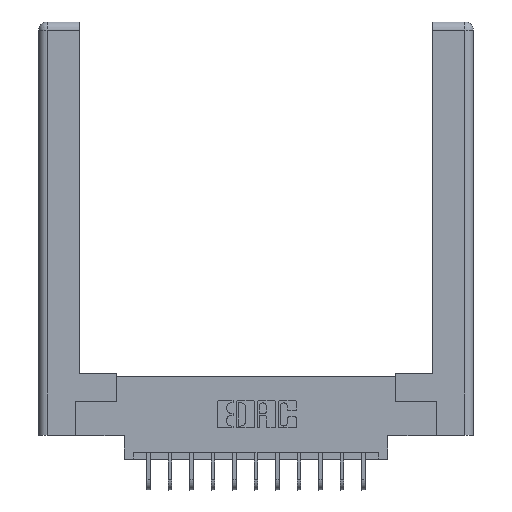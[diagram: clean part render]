
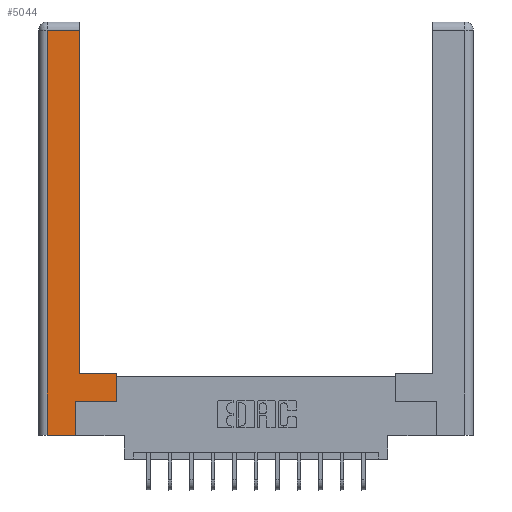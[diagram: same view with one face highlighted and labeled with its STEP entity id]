
A CAD part, top view. The second image highlights one B-rep face of the part: STEP entity #5044.
In plain terms, the highlighted planar face has unit normal (0, 0, 1).
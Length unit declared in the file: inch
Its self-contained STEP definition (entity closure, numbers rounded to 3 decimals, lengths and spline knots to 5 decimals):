
#71 = LINE ( 'NONE', #1686, #12676 ) ;
#264 = EDGE_CURVE ( 'NONE', #10003, #4532, #17100, .T. ) ;
#287 = EDGE_LOOP ( 'NONE', ( #3991, #10321, #2021, #16963, #15825, #12860, #7349, #15462 ) ) ;
#329 = DIRECTION ( 'NONE',  ( 1., 0., 0. ) ) ;
#395 = DIRECTION ( 'NONE',  ( 1., 0., 0. ) ) ;
#688 = VECTOR ( 'NONE', #10674, 39.37008 ) ;
#1391 = CARTESIAN_POINT ( 'NONE',  ( 0.0615, 0., 0. ) ) ;
#1444 = CARTESIAN_POINT ( 'NONE',  ( 0.265, 0.245, 0. ) ) ;
#1686 = CARTESIAN_POINT ( 'NONE',  ( 0.295, 0.45, 0. ) ) ;
#1974 = LINE ( 'NONE', #9517, #12900 ) ;
#2021 = ORIENTED_EDGE ( 'NONE', *, *, #264, .T. ) ;
#2896 = VERTEX_POINT ( 'NONE', #10960 ) ;
#2927 = EDGE_CURVE ( 'NONE', #10829, #9337, #16810, .T. ) ;
#3991 = ORIENTED_EDGE ( 'NONE', *, *, #9519, .T. ) ;
#4105 = VECTOR ( 'NONE', #11520, 39.37008 ) ;
#4425 = CARTESIAN_POINT ( 'NONE',  ( 0.0615, 2.94, 0. ) ) ;
#4426 = AXIS2_PLACEMENT_3D ( 'NONE', #12154, #8090, #5391 ) ;
#4532 = VERTEX_POINT ( 'NONE', #1391 ) ;
#4534 = LINE ( 'NONE', #4994, #4105 ) ;
#4980 = DIRECTION ( 'NONE',  ( -1., 0., 0. ) ) ;
#4994 = CARTESIAN_POINT ( 'NONE',  ( 0.295, 3., 0. ) ) ;
#5044 = ADVANCED_FACE ( 'NONE', ( #5774 ), #13354, .F. ) ;
#5070 = CARTESIAN_POINT ( 'NONE',  ( 0.265, 0.245, 0. ) ) ;
#5391 = DIRECTION ( 'NONE',  ( -1., 0., 0. ) ) ;
#5774 = FACE_OUTER_BOUND ( 'NONE', #287, .T. ) ;
#5861 = CARTESIAN_POINT ( 'NONE',  ( 0.295, 0.45, 0. ) ) ;
#7019 = VECTOR ( 'NONE', #4980, 39.37008 ) ;
#7349 = ORIENTED_EDGE ( 'NONE', *, *, #12414, .T. ) ;
#7910 = EDGE_CURVE ( 'NONE', #4532, #8687, #8053, .T. ) ;
#8053 = LINE ( 'NONE', #9429, #13867 ) ;
#8090 = DIRECTION ( 'NONE',  ( 0., 0., -1. ) ) ;
#8107 = CARTESIAN_POINT ( 'NONE',  ( 0.565, 0.245, 0. ) ) ;
#8336 = EDGE_CURVE ( 'NONE', #2896, #10003, #12626, .T. ) ;
#8687 = VERTEX_POINT ( 'NONE', #15212 ) ;
#8796 = VECTOR ( 'NONE', #10951, 39.37008 ) ;
#9337 = VERTEX_POINT ( 'NONE', #12752 ) ;
#9429 = CARTESIAN_POINT ( 'NONE',  ( 0.265, 0., 0. ) ) ;
#9517 = CARTESIAN_POINT ( 'NONE',  ( 0.565, 0.45, 0. ) ) ;
#9519 = EDGE_CURVE ( 'NONE', #13695, #2896, #4534, .T. ) ;
#9758 = VECTOR ( 'NONE', #395, 39.37008 ) ;
#10003 = VERTEX_POINT ( 'NONE', #4425 ) ;
#10321 = ORIENTED_EDGE ( 'NONE', *, *, #8336, .T. ) ;
#10674 = DIRECTION ( 'NONE',  ( 0., 1., 0. ) ) ;
#10829 = VERTEX_POINT ( 'NONE', #5070 ) ;
#10951 = DIRECTION ( 'NONE',  ( 0., -1., 0. ) ) ;
#10960 = CARTESIAN_POINT ( 'NONE',  ( 0.295, 2.94, 0. ) ) ;
#11065 = CARTESIAN_POINT ( 'NONE',  ( 0.0615, 0., 0. ) ) ;
#11443 = VERTEX_POINT ( 'NONE', #13850 ) ;
#11520 = DIRECTION ( 'NONE',  ( 0., 1., 0. ) ) ;
#12154 = CARTESIAN_POINT ( 'NONE',  ( 0., 0., 0. ) ) ;
#12233 = DIRECTION ( 'NONE',  ( -1., 0., 0. ) ) ;
#12414 = EDGE_CURVE ( 'NONE', #9337, #11443, #1974, .T. ) ;
#12626 = LINE ( 'NONE', #14305, #7019 ) ;
#12676 = VECTOR ( 'NONE', #12233, 39.37008 ) ;
#12752 = CARTESIAN_POINT ( 'NONE',  ( 0.565, 0.245, 0. ) ) ;
#12860 = ORIENTED_EDGE ( 'NONE', *, *, #2927, .T. ) ;
#12900 = VECTOR ( 'NONE', #14870, 39.37008 ) ;
#13077 = EDGE_CURVE ( 'NONE', #11443, #13695, #71, .T. ) ;
#13354 = PLANE ( 'NONE',  #4426 ) ;
#13695 = VERTEX_POINT ( 'NONE', #5861 ) ;
#13850 = CARTESIAN_POINT ( 'NONE',  ( 0.565, 0.45, 0. ) ) ;
#13867 = VECTOR ( 'NONE', #329, 39.37008 ) ;
#14305 = CARTESIAN_POINT ( 'NONE',  ( 0.0615, 2.94, 0. ) ) ;
#14537 = LINE ( 'NONE', #1444, #688 ) ;
#14870 = DIRECTION ( 'NONE',  ( 0., 1., 0. ) ) ;
#15212 = CARTESIAN_POINT ( 'NONE',  ( 0.265, 0., 0. ) ) ;
#15462 = ORIENTED_EDGE ( 'NONE', *, *, #13077, .T. ) ;
#15825 = ORIENTED_EDGE ( 'NONE', *, *, #16899, .T. ) ;
#16810 = LINE ( 'NONE', #8107, #9758 ) ;
#16899 = EDGE_CURVE ( 'NONE', #8687, #10829, #14537, .T. ) ;
#16963 = ORIENTED_EDGE ( 'NONE', *, *, #7910, .T. ) ;
#17100 = LINE ( 'NONE', #11065, #8796 ) ;
